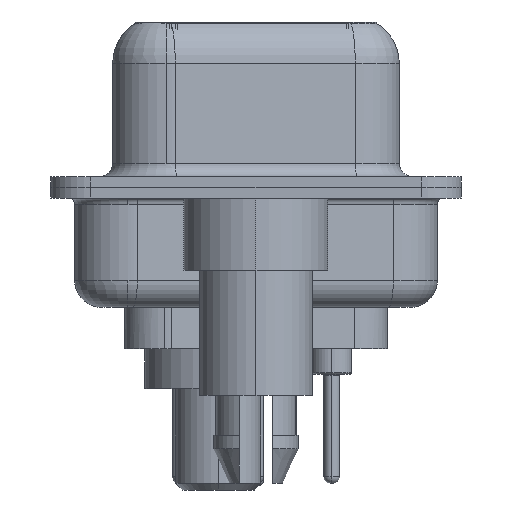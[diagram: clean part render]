
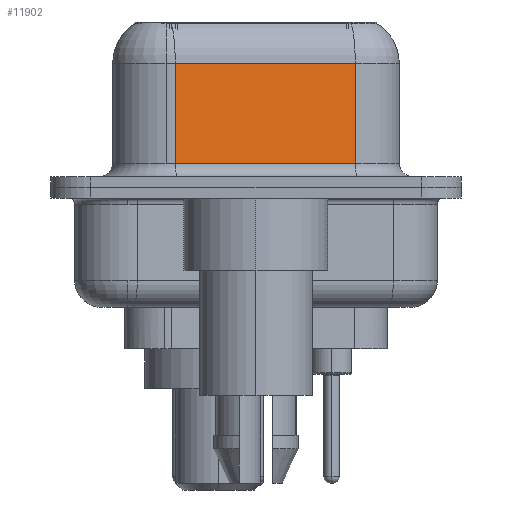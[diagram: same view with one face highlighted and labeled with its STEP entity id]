
A CAD part, left-side view. The second image highlights one B-rep face of the part: STEP entity #11902.
In plain terms, the highlighted planar face has unit normal (-0.985, -0.174, 0).
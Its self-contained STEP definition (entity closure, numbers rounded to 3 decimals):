
#242 = CARTESIAN_POINT ( 'NONE',  ( 5.621, -3.722, 0.9 ) ) ;
#1335 = VERTEX_POINT ( 'NONE', #25369 ) ;
#1656 = LINE ( 'NONE', #16833, #33636 ) ;
#2477 = DIRECTION ( 'NONE',  ( 0.174, -0.985, 0. ) ) ;
#3765 = DIRECTION ( 'NONE',  ( 0., 0., -1. ) ) ;
#3780 = CARTESIAN_POINT ( 'NONE',  ( 5.621, -3.722, 6.4 ) ) ;
#4834 = CARTESIAN_POINT ( 'NONE',  ( 5.621, -3.722, 4.65 ) ) ;
#5759 = ORIENTED_EDGE ( 'NONE', *, *, #6777, .T. ) ;
#6514 = CARTESIAN_POINT ( 'NONE',  ( 4.43, 3.028, 6.4 ) ) ;
#6777 = EDGE_CURVE ( 'NONE', #12198, #1335, #1656, .T. ) ;
#8620 = FACE_OUTER_BOUND ( 'NONE', #25274, .T. ) ;
#9308 = PLANE ( 'NONE',  #11519 ) ;
#10387 = CARTESIAN_POINT ( 'NONE',  ( 5.621, -3.722, 0.9 ) ) ;
#11519 = AXIS2_PLACEMENT_3D ( 'NONE', #3780, #11825, #17386 ) ;
#11646 = LINE ( 'NONE', #6514, #24835 ) ;
#11825 = DIRECTION ( 'NONE',  ( 0.985, 0.174, 0. ) ) ;
#11902 = ADVANCED_FACE ( 'NONE', ( #8620 ), #9308, .F. ) ;
#12198 = VERTEX_POINT ( 'NONE', #4834 ) ;
#12489 = EDGE_CURVE ( 'NONE', #12198, #17704, #32871, .T. ) ;
#12738 = VERTEX_POINT ( 'NONE', #13076 ) ;
#13076 = CARTESIAN_POINT ( 'NONE',  ( 4.43, 3.028, 0.9 ) ) ;
#15848 = ORIENTED_EDGE ( 'NONE', *, *, #30266, .T. ) ;
#16833 = CARTESIAN_POINT ( 'NONE',  ( 5.621, -3.722, 4.65 ) ) ;
#17386 = DIRECTION ( 'NONE',  ( -0.174, 0.985, 0. ) ) ;
#17704 = VERTEX_POINT ( 'NONE', #242 ) ;
#19448 = LINE ( 'NONE', #10387, #29670 ) ;
#20308 = EDGE_CURVE ( 'NONE', #12738, #17704, #19448, .T. ) ;
#20459 = DIRECTION ( 'NONE',  ( 0., 0., -1. ) ) ;
#20975 = ORIENTED_EDGE ( 'NONE', *, *, #12489, .F. ) ;
#24335 = ORIENTED_EDGE ( 'NONE', *, *, #20308, .T. ) ;
#24835 = VECTOR ( 'NONE', #3765, 1000. ) ;
#25274 = EDGE_LOOP ( 'NONE', ( #20975, #5759, #15848, #24335 ) ) ;
#25369 = CARTESIAN_POINT ( 'NONE',  ( 4.43, 3.028, 4.65 ) ) ;
#29670 = VECTOR ( 'NONE', #2477, 1000. ) ;
#30266 = EDGE_CURVE ( 'NONE', #1335, #12738, #11646, .T. ) ;
#30941 = CARTESIAN_POINT ( 'NONE',  ( 5.621, -3.722, 6.4 ) ) ;
#32691 = DIRECTION ( 'NONE',  ( -0.174, 0.985, 0. ) ) ;
#32871 = LINE ( 'NONE', #30941, #34579 ) ;
#33636 = VECTOR ( 'NONE', #32691, 1000. ) ;
#34579 = VECTOR ( 'NONE', #20459, 1000. ) ;
